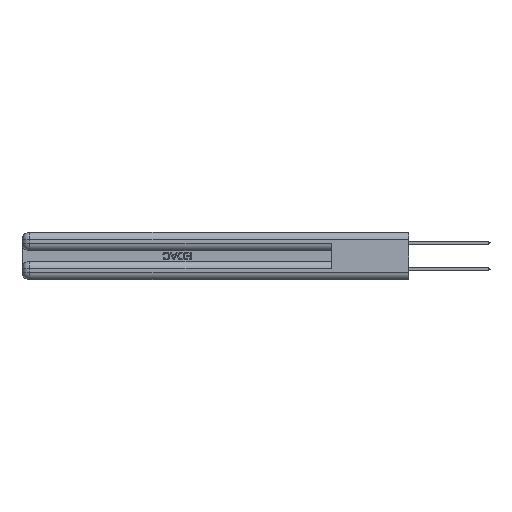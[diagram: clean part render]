
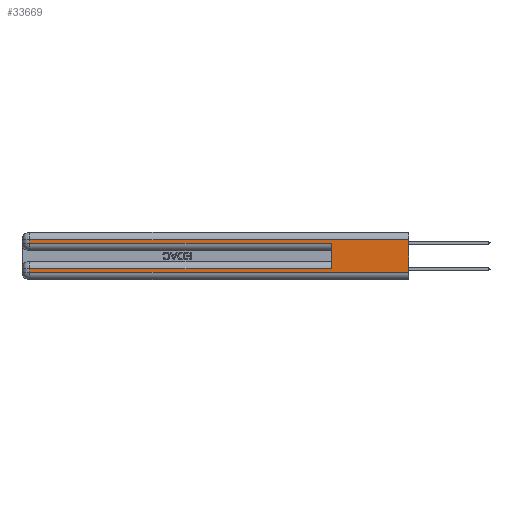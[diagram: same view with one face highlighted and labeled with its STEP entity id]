
A CAD part, left-side view. The second image highlights one B-rep face of the part: STEP entity #33669.
In plain terms, the highlighted planar face has unit normal (-1, 0, 0).
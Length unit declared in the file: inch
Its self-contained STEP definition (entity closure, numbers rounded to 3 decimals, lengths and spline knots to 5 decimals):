
#430 = ORIENTED_EDGE ( 'NONE', *, *, #11151, .T. ) ;
#1566 = DIRECTION ( 'NONE',  ( 0., 0., -1. ) ) ;
#3019 = LINE ( 'NONE', #43372, #42597 ) ;
#3112 = VECTOR ( 'NONE', #48036, 39.37008 ) ;
#4130 = EDGE_CURVE ( 'NONE', #6249, #16711, #19663, .T. ) ;
#4148 = ORIENTED_EDGE ( 'NONE', *, *, #24625, .T. ) ;
#4896 = LINE ( 'NONE', #19814, #24670 ) ;
#5277 = CARTESIAN_POINT ( 'NONE',  ( 0., 0., 0.31 ) ) ;
#6249 = VERTEX_POINT ( 'NONE', #11491 ) ;
#7544 = AXIS2_PLACEMENT_3D ( 'NONE', #22161, #49863, #26157 ) ;
#7956 = DIRECTION ( 'NONE',  ( 0., 0., 1. ) ) ;
#11145 = CARTESIAN_POINT ( 'NONE',  ( 0., 0., 0.06 ) ) ;
#11151 = EDGE_CURVE ( 'NONE', #11950, #18032, #37755, .T. ) ;
#11491 = CARTESIAN_POINT ( 'NONE',  ( 0., 0.6, 0.085 ) ) ;
#11950 = VERTEX_POINT ( 'NONE', #35155 ) ;
#12248 = ORIENTED_EDGE ( 'NONE', *, *, #4130, .T. ) ;
#12842 = ORIENTED_EDGE ( 'NONE', *, *, #22347, .T. ) ;
#14175 = VERTEX_POINT ( 'NONE', #25152 ) ;
#15115 = DIRECTION ( 'NONE',  ( 0., -1., 0. ) ) ;
#16711 = VERTEX_POINT ( 'NONE', #48589 ) ;
#18032 = VERTEX_POINT ( 'NONE', #25125 ) ;
#18236 = PLANE ( 'NONE',  #7544 ) ;
#18320 = LINE ( 'NONE', #33027, #28828 ) ;
#18867 = FACE_OUTER_BOUND ( 'NONE', #19508, .T. ) ;
#19508 = EDGE_LOOP ( 'NONE', ( #22022, #12842, #48027, #430, #31967, #12248, #4148, #46186 ) ) ;
#19663 = LINE ( 'NONE', #33395, #47346 ) ;
#19814 = CARTESIAN_POINT ( 'NONE',  ( 0., 0., 0.37 ) ) ;
#21664 = LINE ( 'NONE', #50429, #41467 ) ;
#22022 = ORIENTED_EDGE ( 'NONE', *, *, #40913, .F. ) ;
#22161 = CARTESIAN_POINT ( 'NONE',  ( 0., 0., 0.37 ) ) ;
#22347 = EDGE_CURVE ( 'NONE', #41122, #25710, #45163, .T. ) ;
#22778 = LINE ( 'NONE', #11145, #42609 ) ;
#23938 = EDGE_CURVE ( 'NONE', #14175, #45521, #22778, .T. ) ;
#24625 = EDGE_CURVE ( 'NONE', #16711, #14175, #21664, .T. ) ;
#24670 = VECTOR ( 'NONE', #27773, 39.37008 ) ;
#25025 = CARTESIAN_POINT ( 'NONE',  ( 0., 0., 0.285 ) ) ;
#25125 = CARTESIAN_POINT ( 'NONE',  ( 0., 0.6, 0.285 ) ) ;
#25152 = CARTESIAN_POINT ( 'NONE',  ( 0., 2.94, 0.06 ) ) ;
#25710 = VERTEX_POINT ( 'NONE', #42359 ) ;
#26157 = DIRECTION ( 'NONE',  ( 0., 0., -1. ) ) ;
#27773 = DIRECTION ( 'NONE',  ( 0., 0., -1. ) ) ;
#28494 = VECTOR ( 'NONE', #48710, 39.37008 ) ;
#28828 = VECTOR ( 'NONE', #1566, 39.37008 ) ;
#30635 = EDGE_CURVE ( 'NONE', #6249, #18032, #3019, .T. ) ;
#30847 = CARTESIAN_POINT ( 'NONE',  ( 0., 0., 0.06 ) ) ;
#31967 = ORIENTED_EDGE ( 'NONE', *, *, #30635, .F. ) ;
#32305 = EDGE_CURVE ( 'NONE', #25710, #11950, #18320, .T. ) ;
#32322 = CARTESIAN_POINT ( 'NONE',  ( 0., 0., 0.31 ) ) ;
#33027 = CARTESIAN_POINT ( 'NONE',  ( 0., 2.94, 0.37 ) ) ;
#33395 = CARTESIAN_POINT ( 'NONE',  ( 0., 0., 0.085 ) ) ;
#33669 = ADVANCED_FACE ( 'NONE', ( #18867 ), #18236, .F. ) ;
#34695 = DIRECTION ( 'NONE',  ( 0., 0., -1. ) ) ;
#35155 = CARTESIAN_POINT ( 'NONE',  ( 0., 2.94, 0.285 ) ) ;
#37341 = DIRECTION ( 'NONE',  ( 0., 1., 0. ) ) ;
#37755 = LINE ( 'NONE', #25025, #28494 ) ;
#40913 = EDGE_CURVE ( 'NONE', #41122, #45521, #4896, .T. ) ;
#41122 = VERTEX_POINT ( 'NONE', #5277 ) ;
#41467 = VECTOR ( 'NONE', #34695, 39.37008 ) ;
#42359 = CARTESIAN_POINT ( 'NONE',  ( 0., 2.94, 0.31 ) ) ;
#42597 = VECTOR ( 'NONE', #7956, 39.37008 ) ;
#42609 = VECTOR ( 'NONE', #15115, 39.37008 ) ;
#43372 = CARTESIAN_POINT ( 'NONE',  ( 0., 0.6, 0.145 ) ) ;
#45163 = LINE ( 'NONE', #32322, #3112 ) ;
#45521 = VERTEX_POINT ( 'NONE', #30847 ) ;
#46186 = ORIENTED_EDGE ( 'NONE', *, *, #23938, .T. ) ;
#47346 = VECTOR ( 'NONE', #37341, 39.37008 ) ;
#48027 = ORIENTED_EDGE ( 'NONE', *, *, #32305, .T. ) ;
#48036 = DIRECTION ( 'NONE',  ( 0., 1., 0. ) ) ;
#48589 = CARTESIAN_POINT ( 'NONE',  ( 0., 2.94, 0.085 ) ) ;
#48710 = DIRECTION ( 'NONE',  ( 0., -1., 0. ) ) ;
#49863 = DIRECTION ( 'NONE',  ( 1., 0., 0. ) ) ;
#50429 = CARTESIAN_POINT ( 'NONE',  ( 0., 2.94, 0.37 ) ) ;
